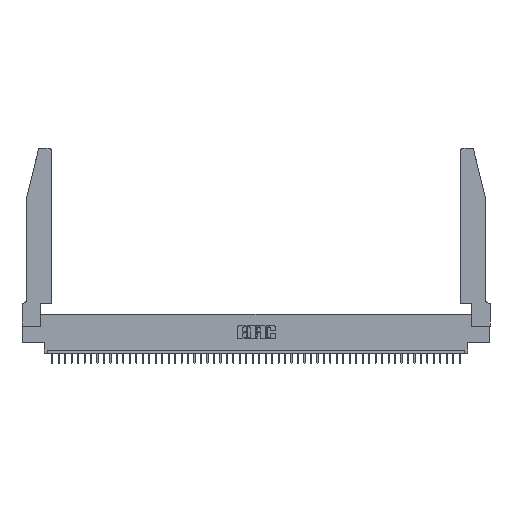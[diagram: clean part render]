
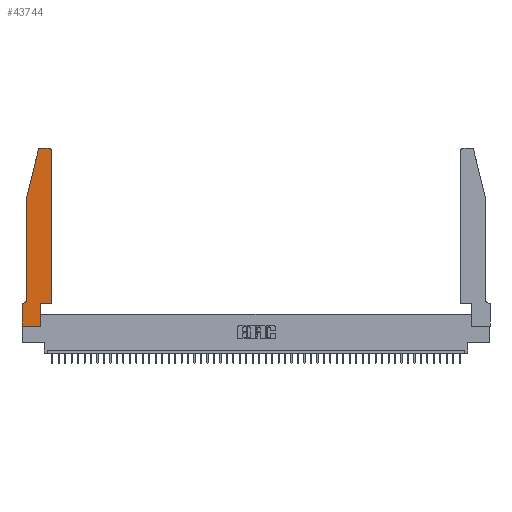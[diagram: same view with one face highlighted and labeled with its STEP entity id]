
A CAD part, top view. The second image highlights one B-rep face of the part: STEP entity #43744.
In plain terms, the highlighted planar face has unit normal (0, 0, 1).
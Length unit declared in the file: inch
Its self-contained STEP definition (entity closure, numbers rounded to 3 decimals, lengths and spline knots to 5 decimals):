
#396 = LINE ( 'NONE', #19832, #19753 ) ;
#1595 = CARTESIAN_POINT ( 'NONE',  ( 0.4205, 2.72, 0.37 ) ) ;
#1693 = ORIENTED_EDGE ( 'NONE', *, *, #14939, .T. ) ;
#3761 = ORIENTED_EDGE ( 'NONE', *, *, #25677, .T. ) ;
#3791 = ORIENTED_EDGE ( 'NONE', *, *, #45246, .T. ) ;
#3859 = DIRECTION ( 'NONE',  ( 0., 0., 1. ) ) ;
#4141 = EDGE_CURVE ( 'NONE', #46838, #8846, #19797, .T. ) ;
#4340 = DIRECTION ( 'NONE',  ( -1., 0., 0. ) ) ;
#4661 = EDGE_CURVE ( 'NONE', #46182, #40318, #15505, .T. ) ;
#4851 = LINE ( 'NONE', #13629, #30885 ) ;
#6824 = CARTESIAN_POINT ( 'NONE',  ( 0.25487, 2.72718, 0.37 ) ) ;
#6966 = VECTOR ( 'NONE', #40497, 39.37008 ) ;
#8017 = CIRCLE ( 'NONE', #40839, 0.03 ) ;
#8187 = CIRCLE ( 'NONE', #27523, 0.03 ) ;
#8217 = ORIENTED_EDGE ( 'NONE', *, *, #41332, .T. ) ;
#8326 = DIRECTION ( 'NONE',  ( 1., 0., 0. ) ) ;
#8547 = DIRECTION ( 'NONE',  ( 1., 0., 0. ) ) ;
#8571 = ORIENTED_EDGE ( 'NONE', *, *, #31544, .T. ) ;
#8706 = ORIENTED_EDGE ( 'NONE', *, *, #12408, .T. ) ;
#8846 = VERTEX_POINT ( 'NONE', #11447 ) ;
#9513 = CARTESIAN_POINT ( 'NONE',  ( 0., 0., 0.37 ) ) ;
#10483 = VECTOR ( 'NONE', #15760, 39.37008 ) ;
#10899 = VERTEX_POINT ( 'NONE', #37961 ) ;
#11183 = CARTESIAN_POINT ( 'NONE',  ( 0.284, 2.75, 0.37 ) ) ;
#11447 = CARTESIAN_POINT ( 'NONE',  ( 0., 0.35, 0.37 ) ) ;
#12408 = EDGE_CURVE ( 'NONE', #37225, #35838, #396, .T. ) ;
#12417 = ORIENTED_EDGE ( 'NONE', *, *, #33711, .T. ) ;
#12500 = ORIENTED_EDGE ( 'NONE', *, *, #4661, .T. ) ;
#12894 = PLANE ( 'NONE',  #28391 ) ;
#13138 = DIRECTION ( 'NONE',  ( 0., 1., 0. ) ) ;
#13470 = EDGE_CURVE ( 'NONE', #8846, #17785, #17235, .T. ) ;
#13629 = CARTESIAN_POINT ( 'NONE',  ( 0., 0., 0.37 ) ) ;
#14418 = ORIENTED_EDGE ( 'NONE', *, *, #14862, .T. ) ;
#14695 = LINE ( 'NONE', #31192, #10483 ) ;
#14862 = EDGE_CURVE ( 'NONE', #40318, #46838, #28657, .T. ) ;
#14939 = EDGE_CURVE ( 'NONE', #34818, #34634, #8017, .T. ) ;
#15505 = LINE ( 'NONE', #38702, #47003 ) ;
#15760 = DIRECTION ( 'NONE',  ( -1., 0., 0. ) ) ;
#16231 = FACE_OUTER_BOUND ( 'NONE', #38110, .T. ) ;
#16271 = DIRECTION ( 'NONE',  ( 1., 0., 0. ) ) ;
#17235 = LINE ( 'NONE', #9513, #6966 ) ;
#17785 = VERTEX_POINT ( 'NONE', #22080 ) ;
#18005 = VERTEX_POINT ( 'NONE', #20477 ) ;
#18486 = LINE ( 'NONE', #33125, #46961 ) ;
#18845 = ORIENTED_EDGE ( 'NONE', *, *, #4141, .T. ) ;
#19339 = DIRECTION ( 'NONE',  ( 0., 0., -1. ) ) ;
#19406 = DIRECTION ( 'NONE',  ( -0.239, -0.971, 0. ) ) ;
#19450 = CARTESIAN_POINT ( 'NONE',  ( 0.0755, 2., 0.37 ) ) ;
#19562 = CARTESIAN_POINT ( 'NONE',  ( 0.0055, 0.35, 0.37 ) ) ;
#19753 = VECTOR ( 'NONE', #8326, 39.37008 ) ;
#19797 = LINE ( 'NONE', #47141, #47053 ) ;
#19832 = CARTESIAN_POINT ( 'NONE',  ( 0.4505, 0.35, 0.37 ) ) ;
#19914 = CARTESIAN_POINT ( 'NONE',  ( 0.0755, 2., 0.37 ) ) ;
#20068 = AXIS2_PLACEMENT_3D ( 'NONE', #23399, #19339, #49831 ) ;
#20477 = CARTESIAN_POINT ( 'NONE',  ( 0.4205, 2.75, 0.37 ) ) ;
#20891 = DIRECTION ( 'NONE',  ( 1., 0., 0. ) ) ;
#21079 = CARTESIAN_POINT ( 'NONE',  ( 0.4505, 0.35, 0.37 ) ) ;
#22080 = CARTESIAN_POINT ( 'NONE',  ( 0., 0., 0.37 ) ) ;
#22181 = LINE ( 'NONE', #46584, #31279 ) ;
#23399 = CARTESIAN_POINT ( 'NONE',  ( 0.0055, 0.42, 0.37 ) ) ;
#24072 = CARTESIAN_POINT ( 'NONE',  ( 0., 0.35, 0.37 ) ) ;
#24397 = DIRECTION ( 'NONE',  ( 0., 0., 1. ) ) ;
#24449 = DIRECTION ( 'NONE',  ( 0., 0., 1. ) ) ;
#25677 = EDGE_CURVE ( 'NONE', #10899, #37225, #22181, .T. ) ;
#26412 = DIRECTION ( 'NONE',  ( 0., -1., 0. ) ) ;
#27051 = CARTESIAN_POINT ( 'NONE',  ( 0.284, 2.72, 0.37 ) ) ;
#27523 = AXIS2_PLACEMENT_3D ( 'NONE', #1595, #24449, #35978 ) ;
#28391 = AXIS2_PLACEMENT_3D ( 'NONE', #24072, #24397, #16271 ) ;
#28657 = CIRCLE ( 'NONE', #20068, 0.07 ) ;
#29285 = VECTOR ( 'NONE', #19406, 39.37008 ) ;
#30885 = VECTOR ( 'NONE', #20891, 39.37008 ) ;
#31192 = CARTESIAN_POINT ( 'NONE',  ( 0.2605, 2.75, 0.37 ) ) ;
#31279 = VECTOR ( 'NONE', #42698, 39.37008 ) ;
#31544 = EDGE_CURVE ( 'NONE', #35838, #32894, #18486, .T. ) ;
#32894 = VERTEX_POINT ( 'NONE', #49608 ) ;
#33125 = CARTESIAN_POINT ( 'NONE',  ( 0.4505, 0.35, 0.37 ) ) ;
#33711 = EDGE_CURVE ( 'NONE', #34634, #46182, #35914, .T. ) ;
#34634 = VERTEX_POINT ( 'NONE', #6824 ) ;
#34818 = VERTEX_POINT ( 'NONE', #11183 ) ;
#35838 = VERTEX_POINT ( 'NONE', #21079 ) ;
#35914 = LINE ( 'NONE', #19914, #29285 ) ;
#35978 = DIRECTION ( 'NONE',  ( 1., 0., 0. ) ) ;
#37225 = VERTEX_POINT ( 'NONE', #46973 ) ;
#37961 = CARTESIAN_POINT ( 'NONE',  ( 0.2865, 0., 0.37 ) ) ;
#38110 = EDGE_LOOP ( 'NONE', ( #8217, #1693, #12417, #12500, #14418, #18845, #49993, #43912, #3761, #8706, #8571, #3791 ) ) ;
#38702 = CARTESIAN_POINT ( 'NONE',  ( 0.0755, 2., 0.37 ) ) ;
#40318 = VERTEX_POINT ( 'NONE', #47704 ) ;
#40497 = DIRECTION ( 'NONE',  ( 0., -1., 0. ) ) ;
#40839 = AXIS2_PLACEMENT_3D ( 'NONE', #27051, #3859, #8547 ) ;
#41332 = EDGE_CURVE ( 'NONE', #18005, #34818, #14695, .T. ) ;
#42698 = DIRECTION ( 'NONE',  ( 0., 1., 0. ) ) ;
#43125 = EDGE_CURVE ( 'NONE', #17785, #10899, #4851, .T. ) ;
#43744 = ADVANCED_FACE ( 'NONE', ( #16231 ), #12894, .T. ) ;
#43912 = ORIENTED_EDGE ( 'NONE', *, *, #43125, .T. ) ;
#45246 = EDGE_CURVE ( 'NONE', #32894, #18005, #8187, .T. ) ;
#46182 = VERTEX_POINT ( 'NONE', #19450 ) ;
#46584 = CARTESIAN_POINT ( 'NONE',  ( 0.2865, 0.35, 0.37 ) ) ;
#46838 = VERTEX_POINT ( 'NONE', #19562 ) ;
#46961 = VECTOR ( 'NONE', #13138, 39.37008 ) ;
#46973 = CARTESIAN_POINT ( 'NONE',  ( 0.2865, 0.35, 0.37 ) ) ;
#47003 = VECTOR ( 'NONE', #26412, 39.37008 ) ;
#47053 = VECTOR ( 'NONE', #4340, 39.37008 ) ;
#47141 = CARTESIAN_POINT ( 'NONE',  ( 0.0755, 0.35, 0.37 ) ) ;
#47704 = CARTESIAN_POINT ( 'NONE',  ( 0.0755, 0.42, 0.37 ) ) ;
#49608 = CARTESIAN_POINT ( 'NONE',  ( 0.4505, 2.72, 0.37 ) ) ;
#49831 = DIRECTION ( 'NONE',  ( -1., 0., 0. ) ) ;
#49993 = ORIENTED_EDGE ( 'NONE', *, *, #13470, .T. ) ;
